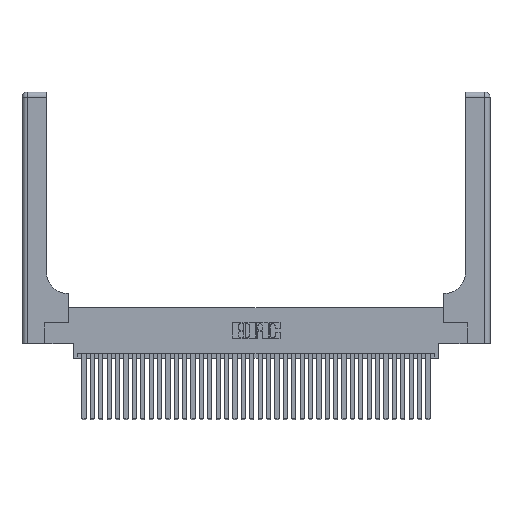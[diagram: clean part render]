
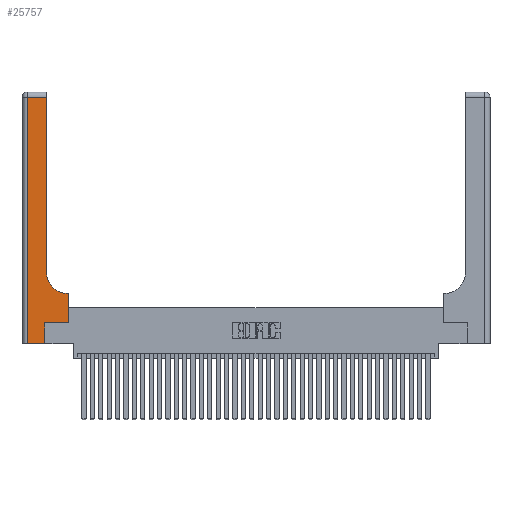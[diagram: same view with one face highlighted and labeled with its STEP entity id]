
A CAD part, top view. The second image highlights one B-rep face of the part: STEP entity #25757.
In plain terms, the highlighted planar face has unit normal (0, 0, 1).
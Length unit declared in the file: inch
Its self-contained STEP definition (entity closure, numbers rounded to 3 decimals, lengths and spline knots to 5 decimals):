
#328 = LINE ( 'NONE', #9663, #15053 ) ;
#1123 = LINE ( 'NONE', #23414, #15832 ) ;
#1633 = AXIS2_PLACEMENT_3D ( 'NONE', #28216, #16487, #37102 ) ;
#1777 = CARTESIAN_POINT ( 'NONE',  ( 0.2915, 0.6, 0.37 ) ) ;
#1817 = VERTEX_POINT ( 'NONE', #33661 ) ;
#2257 = CIRCLE ( 'NONE', #36511, 0.25 ) ;
#2677 = DIRECTION ( 'NONE',  ( 0., -1., 0. ) ) ;
#2702 = ORIENTED_EDGE ( 'NONE', *, *, #11630, .T. ) ;
#3127 = VECTOR ( 'NONE', #22757, 39.37008 ) ;
#3739 = FACE_OUTER_BOUND ( 'NONE', #18380, .T. ) ;
#4755 = DIRECTION ( 'NONE',  ( -1., 0., 0. ) ) ;
#6103 = VECTOR ( 'NONE', #11263, 39.37008 ) ;
#7227 = EDGE_CURVE ( 'NONE', #24396, #34690, #2257, .T. ) ;
#8305 = CARTESIAN_POINT ( 'NONE',  ( 0., 2.94, 0.37 ) ) ;
#8464 = CARTESIAN_POINT ( 'NONE',  ( 0.06, 2.94, 0.37 ) ) ;
#8721 = EDGE_CURVE ( 'NONE', #37221, #37352, #37398, .T. ) ;
#9663 = CARTESIAN_POINT ( 'NONE',  ( 0., 0., 0.37 ) ) ;
#9758 = DIRECTION ( 'NONE',  ( 0., 1., 0. ) ) ;
#11263 = DIRECTION ( 'NONE',  ( -1., 0., 0. ) ) ;
#11496 = VECTOR ( 'NONE', #28488, 39.37008 ) ;
#11586 = CARTESIAN_POINT ( 'NONE',  ( 0.06, 3., 0.37 ) ) ;
#11630 = EDGE_CURVE ( 'NONE', #37041, #24987, #328, .T. ) ;
#12335 = CARTESIAN_POINT ( 'NONE',  ( 0.06, 0., 0.37 ) ) ;
#12907 = VECTOR ( 'NONE', #9758, 39.37008 ) ;
#13256 = ORIENTED_EDGE ( 'NONE', *, *, #8721, .T. ) ;
#13469 = ORIENTED_EDGE ( 'NONE', *, *, #34309, .T. ) ;
#13613 = CARTESIAN_POINT ( 'NONE',  ( 0.5415, 0.85, 0.37 ) ) ;
#15053 = VECTOR ( 'NONE', #30074, 39.37008 ) ;
#15113 = EDGE_CURVE ( 'NONE', #33415, #1817, #1123, .T. ) ;
#15498 = EDGE_CURVE ( 'NONE', #1817, #24396, #28255, .T. ) ;
#15635 = CARTESIAN_POINT ( 'NONE',  ( 0.2915, 3., 0.37 ) ) ;
#15832 = VECTOR ( 'NONE', #26379, 39.37008 ) ;
#16487 = DIRECTION ( 'NONE',  ( 0., 0., -1. ) ) ;
#16536 = DIRECTION ( 'NONE',  ( 1., 0., 0. ) ) ;
#17218 = CARTESIAN_POINT ( 'NONE',  ( 0.269, 0.25, 0.37 ) ) ;
#18090 = VECTOR ( 'NONE', #2677, 39.37008 ) ;
#18380 = EDGE_LOOP ( 'NONE', ( #37632, #13256, #30513, #2702, #31945, #13469, #32959, #25870, #21570 ) ) ;
#18636 = CARTESIAN_POINT ( 'NONE',  ( 0.5585, 0.25, 0.37 ) ) ;
#18859 = CARTESIAN_POINT ( 'NONE',  ( 0.269, 0., 0.37 ) ) ;
#19311 = PLANE ( 'NONE',  #1633 ) ;
#19784 = CARTESIAN_POINT ( 'NONE',  ( 0.269, 0., 0.37 ) ) ;
#21482 = EDGE_CURVE ( 'NONE', #24987, #26810, #26624, .T. ) ;
#21570 = ORIENTED_EDGE ( 'NONE', *, *, #7227, .T. ) ;
#22757 = DIRECTION ( 'NONE',  ( 0., 1., 0. ) ) ;
#23414 = CARTESIAN_POINT ( 'NONE',  ( 0.5585, 0.25, 0.37 ) ) ;
#24084 = CARTESIAN_POINT ( 'NONE',  ( 0.2915, 0.85, 0.37 ) ) ;
#24396 = VERTEX_POINT ( 'NONE', #30994 ) ;
#24628 = EDGE_CURVE ( 'NONE', #37352, #37041, #26858, .T. ) ;
#24987 = VERTEX_POINT ( 'NONE', #18859 ) ;
#25518 = CARTESIAN_POINT ( 'NONE',  ( 0.269, 0.25, 0.37 ) ) ;
#25757 = ADVANCED_FACE ( 'NONE', ( #3739 ), #19311, .F. ) ;
#25870 = ORIENTED_EDGE ( 'NONE', *, *, #15498, .T. ) ;
#26379 = DIRECTION ( 'NONE',  ( 0., 1., 0. ) ) ;
#26408 = VECTOR ( 'NONE', #4755, 39.37008 ) ;
#26624 = LINE ( 'NONE', #19784, #3127 ) ;
#26810 = VERTEX_POINT ( 'NONE', #17218 ) ;
#26858 = LINE ( 'NONE', #11586, #18090 ) ;
#28216 = CARTESIAN_POINT ( 'NONE',  ( 0., 3., 0.37 ) ) ;
#28255 = LINE ( 'NONE', #1777, #26408 ) ;
#28488 = DIRECTION ( 'NONE',  ( 1., 0., 0. ) ) ;
#28541 = LINE ( 'NONE', #15635, #12907 ) ;
#30074 = DIRECTION ( 'NONE',  ( 1., 0., 0. ) ) ;
#30513 = ORIENTED_EDGE ( 'NONE', *, *, #24628, .T. ) ;
#30994 = CARTESIAN_POINT ( 'NONE',  ( 0.5415, 0.6, 0.37 ) ) ;
#31945 = ORIENTED_EDGE ( 'NONE', *, *, #21482, .T. ) ;
#32959 = ORIENTED_EDGE ( 'NONE', *, *, #15113, .T. ) ;
#33415 = VERTEX_POINT ( 'NONE', #18636 ) ;
#33661 = CARTESIAN_POINT ( 'NONE',  ( 0.5585, 0.6, 0.37 ) ) ;
#34067 = EDGE_CURVE ( 'NONE', #34690, #37221, #28541, .T. ) ;
#34202 = DIRECTION ( 'NONE',  ( 0., 0., -1. ) ) ;
#34309 = EDGE_CURVE ( 'NONE', #26810, #33415, #34997, .T. ) ;
#34690 = VERTEX_POINT ( 'NONE', #24084 ) ;
#34997 = LINE ( 'NONE', #25518, #11496 ) ;
#36511 = AXIS2_PLACEMENT_3D ( 'NONE', #13613, #34202, #16536 ) ;
#37041 = VERTEX_POINT ( 'NONE', #12335 ) ;
#37102 = DIRECTION ( 'NONE',  ( -1., 0., 0. ) ) ;
#37221 = VERTEX_POINT ( 'NONE', #37281 ) ;
#37281 = CARTESIAN_POINT ( 'NONE',  ( 0.2915, 2.94, 0.37 ) ) ;
#37352 = VERTEX_POINT ( 'NONE', #8464 ) ;
#37398 = LINE ( 'NONE', #8305, #6103 ) ;
#37632 = ORIENTED_EDGE ( 'NONE', *, *, #34067, .T. ) ;
